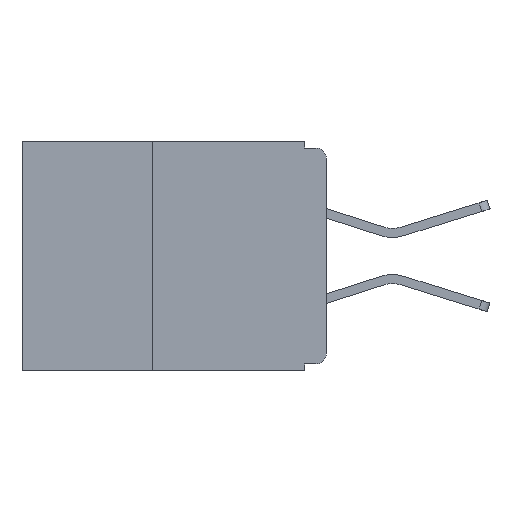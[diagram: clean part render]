
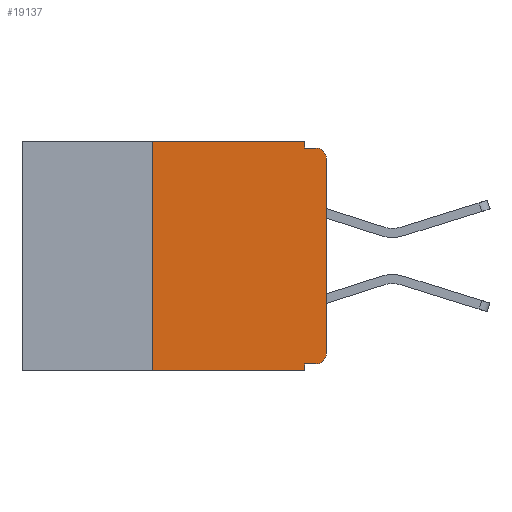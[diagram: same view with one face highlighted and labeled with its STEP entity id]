
A CAD part, left-side view. The second image highlights one B-rep face of the part: STEP entity #19137.
In plain terms, the highlighted planar face has unit normal (-1, 0, 0).
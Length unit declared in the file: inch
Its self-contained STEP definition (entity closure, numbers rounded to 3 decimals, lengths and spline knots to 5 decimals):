
#1090 = CARTESIAN_POINT ( 'NONE',  ( 0., 0., -0.32 ) ) ;
#1217 = ORIENTED_EDGE ( 'NONE', *, *, #17419, .F. ) ;
#1306 = VERTEX_POINT ( 'NONE', #21198 ) ;
#1410 = VECTOR ( 'NONE', #17047, 39.37008 ) ;
#1601 = DIRECTION ( 'NONE',  ( 0., -1., 0. ) ) ;
#1761 = VECTOR ( 'NONE', #1601, 39.37008 ) ;
#1838 = VECTOR ( 'NONE', #10265, 39.37008 ) ;
#1925 = DIRECTION ( 'NONE',  ( 0., -1., 0. ) ) ;
#1980 = VERTEX_POINT ( 'NONE', #20695 ) ;
#2008 = EDGE_CURVE ( 'NONE', #22424, #1306, #5124, .T. ) ;
#2315 = DIRECTION ( 'NONE',  ( 0., 0., 1. ) ) ;
#2600 = ORIENTED_EDGE ( 'NONE', *, *, #17593, .T. ) ;
#3425 = ORIENTED_EDGE ( 'NONE', *, *, #2008, .T. ) ;
#3567 = CARTESIAN_POINT ( 'NONE',  ( 0., 0.015, -0.01 ) ) ;
#3749 = LINE ( 'NONE', #12814, #22613 ) ;
#3924 = CARTESIAN_POINT ( 'NONE',  ( 0., 0.015, -0.025 ) ) ;
#3958 = CARTESIAN_POINT ( 'NONE',  ( 0., 0.031, -0.32 ) ) ;
#4006 = VERTEX_POINT ( 'NONE', #3958 ) ;
#4784 = LINE ( 'NONE', #14161, #23057 ) ;
#4897 = EDGE_LOOP ( 'NONE', ( #3425, #2600, #15512, #14462, #18251, #1217, #22927, #17761, #7578, #20635 ) ) ;
#5124 = LINE ( 'NONE', #7096, #18737 ) ;
#5777 = DIRECTION ( 'NONE',  ( 0., 0., -1. ) ) ;
#6107 = VECTOR ( 'NONE', #11666, 39.37008 ) ;
#6183 = FACE_OUTER_BOUND ( 'NONE', #4897, .T. ) ;
#6362 = DIRECTION ( 'NONE',  ( -1., 0., 0. ) ) ;
#6427 = VERTEX_POINT ( 'NONE', #10885 ) ;
#6651 = LINE ( 'NONE', #18570, #6107 ) ;
#6674 = LINE ( 'NONE', #1090, #1838 ) ;
#6923 = AXIS2_PLACEMENT_3D ( 'NONE', #3924, #16424, #5777 ) ;
#7096 = CARTESIAN_POINT ( 'NONE',  ( 0., 0., 0. ) ) ;
#7578 = ORIENTED_EDGE ( 'NONE', *, *, #9812, .F. ) ;
#7683 = CARTESIAN_POINT ( 'NONE',  ( 0., 0.031, 0. ) ) ;
#7887 = DIRECTION ( 'NONE',  ( 0., 0., -1. ) ) ;
#7896 = CARTESIAN_POINT ( 'NONE',  ( 0., 0.015, -0.32 ) ) ;
#8094 = VERTEX_POINT ( 'NONE', #3567 ) ;
#8300 = CARTESIAN_POINT ( 'NONE',  ( 0., 0., -0.305 ) ) ;
#8410 = EDGE_CURVE ( 'NONE', #11405, #22424, #13513, .T. ) ;
#9812 = EDGE_CURVE ( 'NONE', #11405, #4006, #6674, .T. ) ;
#10265 = DIRECTION ( 'NONE',  ( 0., 1., 0. ) ) ;
#10282 = LINE ( 'NONE', #20559, #1410 ) ;
#10297 = EDGE_CURVE ( 'NONE', #4006, #6427, #6651, .T. ) ;
#10885 = CARTESIAN_POINT ( 'NONE',  ( 0., 0.031, -0.33 ) ) ;
#11405 = VERTEX_POINT ( 'NONE', #7896 ) ;
#11666 = DIRECTION ( 'NONE',  ( 0., 0., -1. ) ) ;
#12161 = EDGE_CURVE ( 'NONE', #1980, #16319, #10282, .T. ) ;
#12237 = AXIS2_PLACEMENT_3D ( 'NONE', #16993, #6362, #18740 ) ;
#12814 = CARTESIAN_POINT ( 'NONE',  ( 0., 0.437, -0.33 ) ) ;
#13513 = CIRCLE ( 'NONE', #12237, 0.015 ) ;
#13851 = CARTESIAN_POINT ( 'NONE',  ( 0., 0.25, -0.33 ) ) ;
#14120 = CARTESIAN_POINT ( 'NONE',  ( 0., 0.031, -0.01 ) ) ;
#14161 = CARTESIAN_POINT ( 'NONE',  ( 0., 0.25, -0.33 ) ) ;
#14227 = CARTESIAN_POINT ( 'NONE',  ( 0., 0., -0.01 ) ) ;
#14462 = ORIENTED_EDGE ( 'NONE', *, *, #18422, .F. ) ;
#15053 = VERTEX_POINT ( 'NONE', #13851 ) ;
#15186 = EDGE_CURVE ( 'NONE', #19352, #8094, #15528, .T. ) ;
#15269 = EDGE_CURVE ( 'NONE', #15053, #6427, #3749, .T. ) ;
#15512 = ORIENTED_EDGE ( 'NONE', *, *, #15186, .F. ) ;
#15528 = LINE ( 'NONE', #14227, #1761 ) ;
#16319 = VERTEX_POINT ( 'NONE', #19984 ) ;
#16424 = DIRECTION ( 'NONE',  ( -1., 0., 0. ) ) ;
#16491 = LINE ( 'NONE', #7683, #17034 ) ;
#16695 = PLANE ( 'NONE',  #21290 ) ;
#16993 = CARTESIAN_POINT ( 'NONE',  ( 0., 0.015, -0.305 ) ) ;
#17034 = VECTOR ( 'NONE', #18238, 39.37008 ) ;
#17047 = DIRECTION ( 'NONE',  ( 0., -1., 0. ) ) ;
#17419 = EDGE_CURVE ( 'NONE', #15053, #1980, #4784, .T. ) ;
#17593 = EDGE_CURVE ( 'NONE', #1306, #8094, #19211, .T. ) ;
#17761 = ORIENTED_EDGE ( 'NONE', *, *, #10297, .F. ) ;
#18238 = DIRECTION ( 'NONE',  ( 0., 0., -1. ) ) ;
#18251 = ORIENTED_EDGE ( 'NONE', *, *, #12161, .F. ) ;
#18422 = EDGE_CURVE ( 'NONE', #16319, #19352, #16491, .T. ) ;
#18437 = DIRECTION ( 'NONE',  ( 1., 0., 0. ) ) ;
#18570 = CARTESIAN_POINT ( 'NONE',  ( 0., 0.031, -0.33 ) ) ;
#18737 = VECTOR ( 'NONE', #2315, 39.37008 ) ;
#18740 = DIRECTION ( 'NONE',  ( 0., 0., -1. ) ) ;
#19137 = ADVANCED_FACE ( 'NONE', ( #6183 ), #16695, .F. ) ;
#19211 = CIRCLE ( 'NONE', #6923, 0.015 ) ;
#19352 = VERTEX_POINT ( 'NONE', #14120 ) ;
#19984 = CARTESIAN_POINT ( 'NONE',  ( 0., 0.031, 0. ) ) ;
#20559 = CARTESIAN_POINT ( 'NONE',  ( 0., 0.437, 0. ) ) ;
#20635 = ORIENTED_EDGE ( 'NONE', *, *, #8410, .T. ) ;
#20695 = CARTESIAN_POINT ( 'NONE',  ( 0., 0.25, 0. ) ) ;
#21198 = CARTESIAN_POINT ( 'NONE',  ( 0., 0., -0.025 ) ) ;
#21290 = AXIS2_PLACEMENT_3D ( 'NONE', #21897, #18437, #7887 ) ;
#21897 = CARTESIAN_POINT ( 'NONE',  ( 0., 0.437, 0. ) ) ;
#22424 = VERTEX_POINT ( 'NONE', #8300 ) ;
#22613 = VECTOR ( 'NONE', #1925, 39.37008 ) ;
#22831 = DIRECTION ( 'NONE',  ( 0., 0., 1. ) ) ;
#22927 = ORIENTED_EDGE ( 'NONE', *, *, #15269, .T. ) ;
#23057 = VECTOR ( 'NONE', #22831, 39.37008 ) ;
